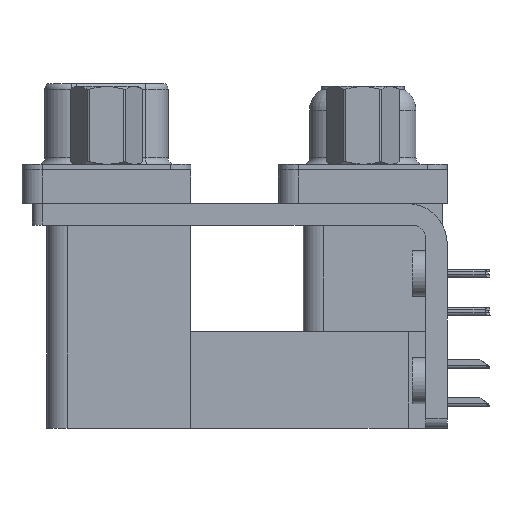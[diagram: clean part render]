
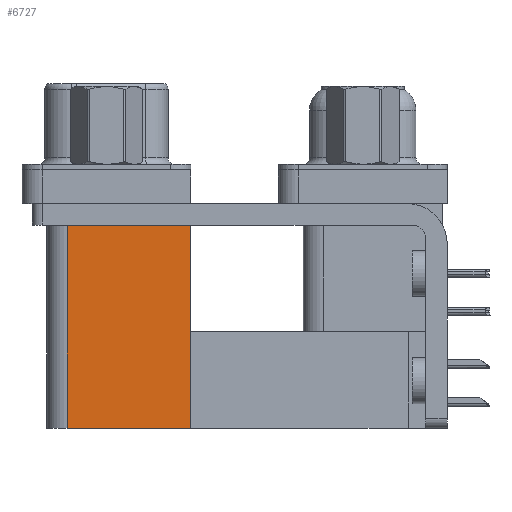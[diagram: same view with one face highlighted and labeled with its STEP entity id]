
A CAD part, left-side view. The second image highlights one B-rep face of the part: STEP entity #6727.
In plain terms, the highlighted planar face has unit normal (-1, 0, 0).
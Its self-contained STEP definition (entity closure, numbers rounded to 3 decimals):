
#1438 = DIRECTION ( 'NONE',  ( 0., 1., 0. ) ) ;
#1574 = EDGE_CURVE ( 'NONE', #30021, #34978, #26224, .T. ) ;
#3566 = EDGE_CURVE ( 'NONE', #34978, #50354, #34065, .T. ) ;
#3930 = ORIENTED_EDGE ( 'NONE', *, *, #1574, .F. ) ;
#5991 = ORIENTED_EDGE ( 'NONE', *, *, #45412, .T. ) ;
#6302 = CARTESIAN_POINT ( 'NONE',  ( 3.765, 21.975, -2.5 ) ) ;
#6346 = CARTESIAN_POINT ( 'NONE',  ( 3.765, 12.775, -19.2 ) ) ;
#6727 = ADVANCED_FACE ( 'NONE', ( #27745 ), #31906, .F. ) ;
#7718 = CARTESIAN_POINT ( 'NONE',  ( 3.765, 12.775, -19.2 ) ) ;
#7733 = VECTOR ( 'NONE', #44882, 1000. ) ;
#9693 = ORIENTED_EDGE ( 'NONE', *, *, #3566, .F. ) ;
#13619 = LINE ( 'NONE', #21423, #49888 ) ;
#17534 = EDGE_LOOP ( 'NONE', ( #32051, #9693, #3930, #5991 ) ) ;
#17654 = DIRECTION ( 'NONE',  ( 0., 1., 0. ) ) ;
#19684 = CARTESIAN_POINT ( 'NONE',  ( 3.765, 21.975, -19.2 ) ) ;
#21423 = CARTESIAN_POINT ( 'NONE',  ( 3.765, 12.775, -2.5 ) ) ;
#22405 = CARTESIAN_POINT ( 'NONE',  ( 3.765, 12.775, -2.5 ) ) ;
#26224 = LINE ( 'NONE', #34010, #37341 ) ;
#27067 = VECTOR ( 'NONE', #49614, 1000. ) ;
#27745 = FACE_OUTER_BOUND ( 'NONE', #17534, .T. ) ;
#29073 = CARTESIAN_POINT ( 'NONE',  ( 3.765, 12.775, -19.2 ) ) ;
#30021 = VERTEX_POINT ( 'NONE', #6346 ) ;
#31480 = VERTEX_POINT ( 'NONE', #22405 ) ;
#31906 = PLANE ( 'NONE',  #34587 ) ;
#32051 = ORIENTED_EDGE ( 'NONE', *, *, #48311, .T. ) ;
#34010 = CARTESIAN_POINT ( 'NONE',  ( 3.765, 12.775, -19.2 ) ) ;
#34065 = LINE ( 'NONE', #37714, #27067 ) ;
#34587 = AXIS2_PLACEMENT_3D ( 'NONE', #7718, #51320, #47432 ) ;
#34978 = VERTEX_POINT ( 'NONE', #19684 ) ;
#37341 = VECTOR ( 'NONE', #17654, 1000. ) ;
#37714 = CARTESIAN_POINT ( 'NONE',  ( 3.765, 21.975, -19.2 ) ) ;
#44882 = DIRECTION ( 'NONE',  ( 0., 0., 1. ) ) ;
#45412 = EDGE_CURVE ( 'NONE', #30021, #31480, #48772, .T. ) ;
#47432 = DIRECTION ( 'NONE',  ( 0., 0., -1. ) ) ;
#48311 = EDGE_CURVE ( 'NONE', #31480, #50354, #13619, .T. ) ;
#48772 = LINE ( 'NONE', #29073, #7733 ) ;
#49614 = DIRECTION ( 'NONE',  ( 0., 0., 1. ) ) ;
#49888 = VECTOR ( 'NONE', #1438, 1000. ) ;
#50354 = VERTEX_POINT ( 'NONE', #6302 ) ;
#51320 = DIRECTION ( 'NONE',  ( 1., 0., 0. ) ) ;
